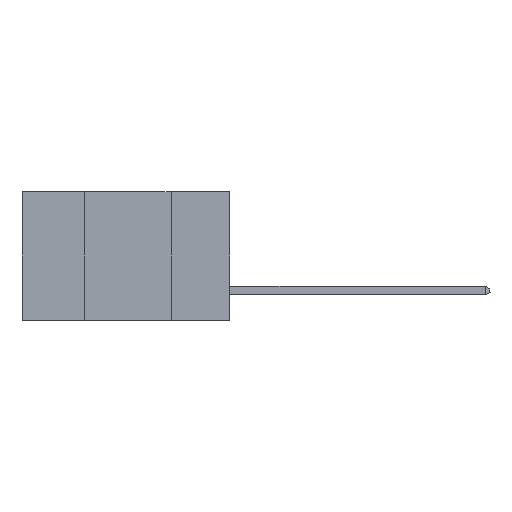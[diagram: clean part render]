
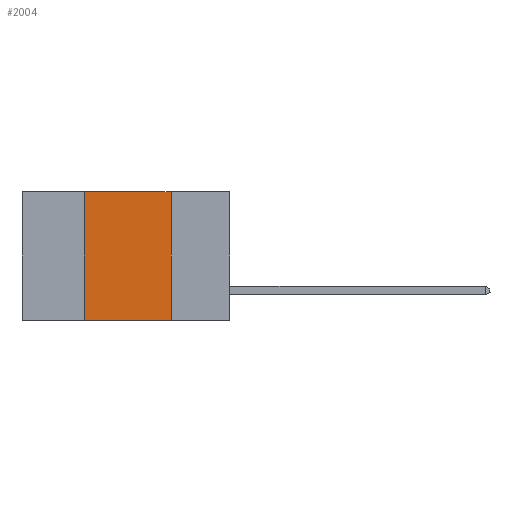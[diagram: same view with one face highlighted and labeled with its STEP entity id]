
A CAD part, left-side view. The second image highlights one B-rep face of the part: STEP entity #2004.
In plain terms, the highlighted planar face has unit normal (-1, 0, 0).
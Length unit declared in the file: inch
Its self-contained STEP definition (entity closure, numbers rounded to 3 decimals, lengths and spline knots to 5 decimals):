
#157 = VECTOR ( 'NONE', #24560, 39.37008 ) ;
#1723 = LINE ( 'NONE', #19178, #12949 ) ;
#2004 = ADVANCED_FACE ( 'NONE', ( #12043 ), #3344, .F. ) ;
#2731 = ORIENTED_EDGE ( 'NONE', *, *, #16552, .T. ) ;
#2930 = VERTEX_POINT ( 'NONE', #3387 ) ;
#3344 = PLANE ( 'NONE',  #21847 ) ;
#3387 = CARTESIAN_POINT ( 'NONE',  ( 0., 0.42, 0. ) ) ;
#4588 = LINE ( 'NONE', #6631, #8364 ) ;
#5452 = EDGE_CURVE ( 'NONE', #28692, #17521, #8494, .T. ) ;
#6631 = CARTESIAN_POINT ( 'NONE',  ( 0., 0.42, 0. ) ) ;
#7048 = DIRECTION ( 'NONE',  ( 0., 0., 1. ) ) ;
#8364 = VECTOR ( 'NONE', #7048, 39.37008 ) ;
#8494 = LINE ( 'NONE', #10807, #17902 ) ;
#10003 = ORIENTED_EDGE ( 'NONE', *, *, #27907, .F. ) ;
#10015 = CARTESIAN_POINT ( 'NONE',  ( 0., 0.6, 0. ) ) ;
#10782 = CARTESIAN_POINT ( 'NONE',  ( 0., 0.42, -0.37 ) ) ;
#10807 = CARTESIAN_POINT ( 'NONE',  ( 0., 0.17, 0. ) ) ;
#11365 = EDGE_CURVE ( 'NONE', #2930, #28692, #24285, .T. ) ;
#12043 = FACE_OUTER_BOUND ( 'NONE', #17819, .T. ) ;
#12949 = VECTOR ( 'NONE', #28031, 39.37008 ) ;
#14378 = DIRECTION ( 'NONE',  ( 0., 0., -1. ) ) ;
#15961 = ORIENTED_EDGE ( 'NONE', *, *, #5452, .F. ) ;
#16552 = EDGE_CURVE ( 'NONE', #28588, #17521, #1723, .T. ) ;
#17358 = DIRECTION ( 'NONE',  ( 0., 0., -1. ) ) ;
#17521 = VERTEX_POINT ( 'NONE', #26458 ) ;
#17819 = EDGE_LOOP ( 'NONE', ( #15961, #25324, #10003, #2731 ) ) ;
#17902 = VECTOR ( 'NONE', #17358, 39.37008 ) ;
#19178 = CARTESIAN_POINT ( 'NONE',  ( 0., 0.6, -0.37 ) ) ;
#20357 = CARTESIAN_POINT ( 'NONE',  ( 0., 0.6, 0. ) ) ;
#21847 = AXIS2_PLACEMENT_3D ( 'NONE', #10015, #24059, #14378 ) ;
#23727 = CARTESIAN_POINT ( 'NONE',  ( 0., 0.17, 0. ) ) ;
#24059 = DIRECTION ( 'NONE',  ( 1., 0., 0. ) ) ;
#24285 = LINE ( 'NONE', #20357, #157 ) ;
#24560 = DIRECTION ( 'NONE',  ( 0., -1., 0. ) ) ;
#25324 = ORIENTED_EDGE ( 'NONE', *, *, #11365, .F. ) ;
#26458 = CARTESIAN_POINT ( 'NONE',  ( 0., 0.17, -0.37 ) ) ;
#27907 = EDGE_CURVE ( 'NONE', #28588, #2930, #4588, .T. ) ;
#28031 = DIRECTION ( 'NONE',  ( 0., -1., 0. ) ) ;
#28588 = VERTEX_POINT ( 'NONE', #10782 ) ;
#28692 = VERTEX_POINT ( 'NONE', #23727 ) ;
